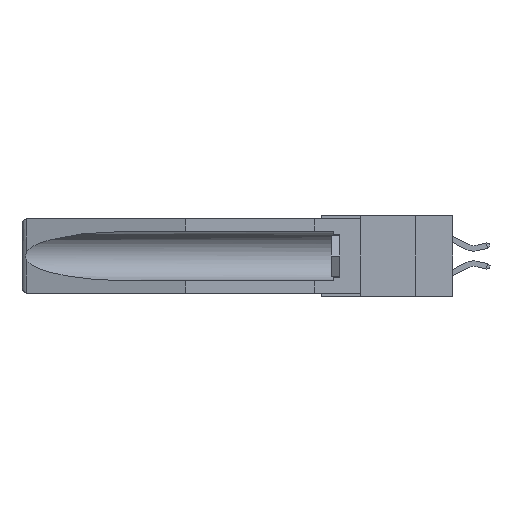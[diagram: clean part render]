
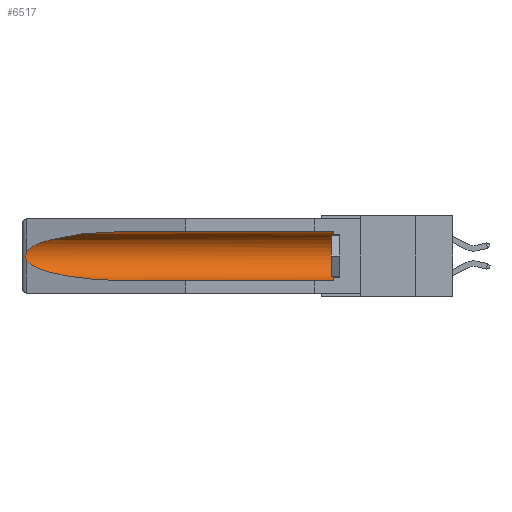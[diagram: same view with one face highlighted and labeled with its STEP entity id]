
A CAD part, left-side view. The second image highlights one B-rep face of the part: STEP entity #6517.
In plain terms, the highlighted cylindrical face has radius 2.857 mm (diameter 5.715 mm), a partial arc.
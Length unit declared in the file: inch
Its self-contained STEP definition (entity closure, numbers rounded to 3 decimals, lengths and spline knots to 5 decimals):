
#45 = CARTESIAN_POINT ( 'NONE',  ( 0.21114, 1.30732, -0.284 ) ) ;
#450 = EDGE_CURVE ( 'NONE', #11515, #12041, #1176, .T. ) ;
#698 = CARTESIAN_POINT ( 'NONE',  ( 0.26537, 1.52718, -0.14972 ) ) ;
#862 = CARTESIAN_POINT ( 'NONE',  ( 0.21114, 1.30732, -0.059 ) ) ;
#1176 = B_SPLINE_CURVE_WITH_KNOTS ( 'NONE', 3,
 ( #698, #27858, #16724, #9852, #1199, #27948, #12034, #16917, #21281, #7804 ),
 .UNSPECIFIED., .F., .F.,
 ( 4, 2, 2, 2, 4 ),
 ( 0., 0.00029, 0.00058, 0.00087, 0.00117 ),
 .UNSPECIFIED. ) ;
#1199 = CARTESIAN_POINT ( 'NONE',  ( 0.2675, 1.53308, -0.16763 ) ) ;
#2073 = EDGE_CURVE ( 'NONE', #7910, #14871, #15263, .T. ) ;
#2398 = CARTESIAN_POINT ( 'NONE',  ( 0.26537, 1.52718, -0.19328 ) ) ;
#2572 = EDGE_CURVE ( 'NONE', #14871, #11515, #8521, .T. ) ;
#2988 = EDGE_CURVE ( 'NONE', #28504, #28722, #11292, .T. ) ;
#3424 = DIRECTION ( 'NONE',  ( 0., 0., 1. ) ) ;
#4425 = DIRECTION ( 'NONE',  ( 0., -1., 0. ) ) ;
#4587 = CARTESIAN_POINT ( 'NONE',  ( 0.26537, 1.52718, -0.19328 ) ) ;
#5753 = CIRCLE ( 'NONE', #22483, 0.1125 ) ;
#6317 =( BOUNDED_CURVE ( )  B_SPLINE_CURVE ( 3, ( #4587, #16048, #45, #18399 ),
 .UNSPECIFIED., .F., .F. ) 
 B_SPLINE_CURVE_WITH_KNOTS ( ( 4, 4 ),
 ( 0.1948, 1.5708 ),
 .UNSPECIFIED. ) 
 CURVE ( )  GEOMETRIC_REPRESENTATION_ITEM ( )  RATIONAL_B_SPLINE_CURVE ( ( 1., 0.848, 0.848, 1. ) ) 
 REPRESENTATION_ITEM ( '' )  );
#6384 = EDGE_LOOP ( 'NONE', ( #16984, #20143, #11763, #26362, #11519, #20725 ) ) ;
#6517 = ADVANCED_FACE ( 'NONE', ( #25218 ), #24889, .F. ) ;
#7804 = CARTESIAN_POINT ( 'NONE',  ( 0.26537, 1.52718, -0.19328 ) ) ;
#7910 = VERTEX_POINT ( 'NONE', #11724 ) ;
#8521 =( BOUNDED_CURVE ( )  B_SPLINE_CURVE ( 3, ( #23233, #862, #14046, #18653 ),
 .UNSPECIFIED., .F., .F. ) 
 B_SPLINE_CURVE_WITH_KNOTS ( ( 4, 4 ),
 ( 4.71239, 6.08839 ),
 .UNSPECIFIED. ) 
 CURVE ( )  GEOMETRIC_REPRESENTATION_ITEM ( )  RATIONAL_B_SPLINE_CURVE ( ( 1., 0.848, 0.848, 1. ) ) 
 REPRESENTATION_ITEM ( '' )  );
#8522 = CARTESIAN_POINT ( 'NONE',  ( 0.155, -0.30754, -0.284 ) ) ;
#9852 = CARTESIAN_POINT ( 'NONE',  ( 0.2673, 1.5327, -0.16383 ) ) ;
#9881 = DIRECTION ( 'NONE',  ( 0., 1., 0. ) ) ;
#10761 = CARTESIAN_POINT ( 'NONE',  ( 0.26537, 1.52718, -0.14972 ) ) ;
#11292 = LINE ( 'NONE', #8522, #28795 ) ;
#11515 = VERTEX_POINT ( 'NONE', #10761 ) ;
#11519 = ORIENTED_EDGE ( 'NONE', *, *, #13188, .T. ) ;
#11710 = VECTOR ( 'NONE', #25456, 39.37008 ) ;
#11724 = CARTESIAN_POINT ( 'NONE',  ( 0.155, 0.126, -0.059 ) ) ;
#11763 = ORIENTED_EDGE ( 'NONE', *, *, #12402, .T. ) ;
#12034 = CARTESIAN_POINT ( 'NONE',  ( 0.2673, 1.53269, -0.17917 ) ) ;
#12041 = VERTEX_POINT ( 'NONE', #2398 ) ;
#12402 = EDGE_CURVE ( 'NONE', #12041, #28722, #6317, .T. ) ;
#12746 = CARTESIAN_POINT ( 'NONE',  ( 0.155, 0.126, -0.284 ) ) ;
#13188 = EDGE_CURVE ( 'NONE', #28504, #7910, #5753, .T. ) ;
#14046 = CARTESIAN_POINT ( 'NONE',  ( 0.25451, 1.48313, -0.09465 ) ) ;
#14871 = VERTEX_POINT ( 'NONE', #17734 ) ;
#15263 = LINE ( 'NONE', #27926, #11710 ) ;
#16048 = CARTESIAN_POINT ( 'NONE',  ( 0.25451, 1.48313, -0.24835 ) ) ;
#16724 = CARTESIAN_POINT ( 'NONE',  ( 0.26654, 1.53092, -0.15636 ) ) ;
#16818 = CARTESIAN_POINT ( 'NONE',  ( 0.155, 1.07973, -0.284 ) ) ;
#16917 = CARTESIAN_POINT ( 'NONE',  ( 0.26655, 1.53094, -0.18657 ) ) ;
#16984 = ORIENTED_EDGE ( 'NONE', *, *, #2572, .T. ) ;
#17183 = AXIS2_PLACEMENT_3D ( 'NONE', #23252, #9881, #3424 ) ;
#17734 = CARTESIAN_POINT ( 'NONE',  ( 0.155, 1.07973, -0.059 ) ) ;
#18399 = CARTESIAN_POINT ( 'NONE',  ( 0.155, 1.07973, -0.284 ) ) ;
#18653 = CARTESIAN_POINT ( 'NONE',  ( 0.26537, 1.52718, -0.14972 ) ) ;
#20143 = ORIENTED_EDGE ( 'NONE', *, *, #450, .T. ) ;
#20725 = ORIENTED_EDGE ( 'NONE', *, *, #2073, .T. ) ;
#21281 = CARTESIAN_POINT ( 'NONE',  ( 0.26597, 1.5296, -0.19026 ) ) ;
#22108 = DIRECTION ( 'NONE',  ( 0., 0., 1. ) ) ;
#22483 = AXIS2_PLACEMENT_3D ( 'NONE', #28716, #4425, #22108 ) ;
#23233 = CARTESIAN_POINT ( 'NONE',  ( 0.155, 1.07973, -0.059 ) ) ;
#23252 = CARTESIAN_POINT ( 'NONE',  ( 0.155, -0.30754, -0.1715 ) ) ;
#24889 = CYLINDRICAL_SURFACE ( 'NONE', #17183, 0.1125 ) ;
#25218 = FACE_OUTER_BOUND ( 'NONE', #6384, .T. ) ;
#25456 = DIRECTION ( 'NONE',  ( 0., 1., 0. ) ) ;
#26362 = ORIENTED_EDGE ( 'NONE', *, *, #2988, .F. ) ;
#27858 = CARTESIAN_POINT ( 'NONE',  ( 0.26597, 1.52961, -0.15275 ) ) ;
#27926 = CARTESIAN_POINT ( 'NONE',  ( 0.155, -0.30754, -0.059 ) ) ;
#27948 = CARTESIAN_POINT ( 'NONE',  ( 0.2675, 1.53308, -0.17534 ) ) ;
#28504 = VERTEX_POINT ( 'NONE', #12746 ) ;
#28716 = CARTESIAN_POINT ( 'NONE',  ( 0.155, 0.126, -0.1715 ) ) ;
#28722 = VERTEX_POINT ( 'NONE', #16818 ) ;
#28744 = DIRECTION ( 'NONE',  ( 0., 1., 0. ) ) ;
#28795 = VECTOR ( 'NONE', #28744, 39.37008 ) ;
